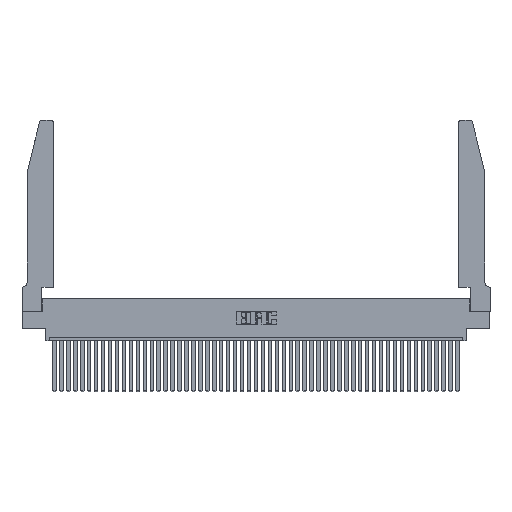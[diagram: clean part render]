
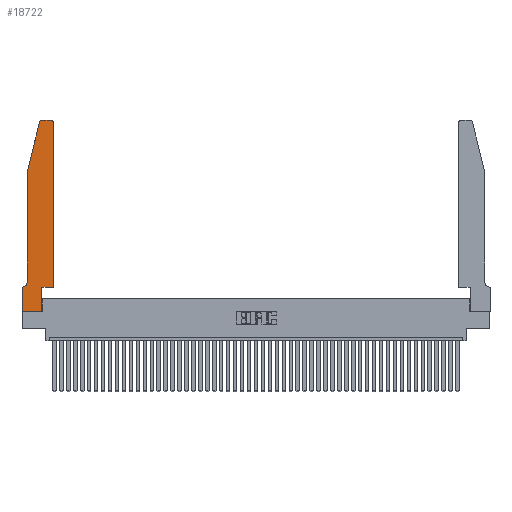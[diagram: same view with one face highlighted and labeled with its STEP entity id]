
A CAD part, top view. The second image highlights one B-rep face of the part: STEP entity #18722.
In plain terms, the highlighted planar face has unit normal (0, 0, 1).
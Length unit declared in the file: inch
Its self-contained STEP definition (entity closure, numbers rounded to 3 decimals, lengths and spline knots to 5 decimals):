
#283 = ORIENTED_EDGE ( 'NONE', *, *, #8491, .T. ) ;
#313 = CIRCLE ( 'NONE', #10665, 0.03 ) ;
#871 = DIRECTION ( 'NONE',  ( 0., 1., 0. ) ) ;
#1090 = AXIS2_PLACEMENT_3D ( 'NONE', #26872, #19271, #1280 ) ;
#1280 = DIRECTION ( 'NONE',  ( -1., 0., 0. ) ) ;
#1536 = CARTESIAN_POINT ( 'NONE',  ( 0.284, 2.72, 0.37 ) ) ;
#1584 = CARTESIAN_POINT ( 'NONE',  ( 0.0755, 2., 0.37 ) ) ;
#2343 = VERTEX_POINT ( 'NONE', #5293 ) ;
#2633 = LINE ( 'NONE', #21457, #19011 ) ;
#3047 = VECTOR ( 'NONE', #44415, 39.37008 ) ;
#3525 = CARTESIAN_POINT ( 'NONE',  ( 0.4505, 0.35, 0.37 ) ) ;
#4507 = EDGE_CURVE ( 'NONE', #11555, #20846, #2633, .T. ) ;
#5060 = DIRECTION ( 'NONE',  ( 1., 0., 0. ) ) ;
#5293 = CARTESIAN_POINT ( 'NONE',  ( 0.2865, 0.35, 0.37 ) ) ;
#5360 = ORIENTED_EDGE ( 'NONE', *, *, #40942, .T. ) ;
#5952 = EDGE_CURVE ( 'NONE', #9379, #37491, #46015, .T. ) ;
#7135 = CARTESIAN_POINT ( 'NONE',  ( 0.0755, 0.42, 0.37 ) ) ;
#7204 = CARTESIAN_POINT ( 'NONE',  ( 0.4505, 0.35, 0.37 ) ) ;
#7274 = EDGE_CURVE ( 'NONE', #20846, #2343, #31733, .T. ) ;
#7823 = VECTOR ( 'NONE', #12005, 39.37008 ) ;
#8034 = CARTESIAN_POINT ( 'NONE',  ( 0.0755, 2., 0.37 ) ) ;
#8142 = LINE ( 'NONE', #18958, #3047 ) ;
#8491 = EDGE_CURVE ( 'NONE', #11571, #30345, #36037, .T. ) ;
#9094 = LINE ( 'NONE', #40212, #46396 ) ;
#9171 = VERTEX_POINT ( 'NONE', #32146 ) ;
#9379 = VERTEX_POINT ( 'NONE', #26579 ) ;
#10449 = EDGE_CURVE ( 'NONE', #13111, #12483, #8142, .T. ) ;
#10665 = AXIS2_PLACEMENT_3D ( 'NONE', #25109, #39788, #43421 ) ;
#11555 = VERTEX_POINT ( 'NONE', #32080 ) ;
#11571 = VERTEX_POINT ( 'NONE', #43424 ) ;
#12005 = DIRECTION ( 'NONE',  ( 0., -1., 0. ) ) ;
#12114 = VECTOR ( 'NONE', #27587, 39.37008 ) ;
#12470 = PLANE ( 'NONE',  #38054 ) ;
#12483 = VERTEX_POINT ( 'NONE', #39222 ) ;
#12697 = LINE ( 'NONE', #19824, #12114 ) ;
#12768 = CARTESIAN_POINT ( 'NONE',  ( 0.284, 2.75, 0.37 ) ) ;
#12787 = ORIENTED_EDGE ( 'NONE', *, *, #10449, .T. ) ;
#13067 = VERTEX_POINT ( 'NONE', #31155 ) ;
#13111 = VERTEX_POINT ( 'NONE', #13577 ) ;
#13577 = CARTESIAN_POINT ( 'NONE',  ( 0.0055, 0.35, 0.37 ) ) ;
#15558 = LINE ( 'NONE', #8034, #38167 ) ;
#17990 = DIRECTION ( 'NONE',  ( 1., 0., 0. ) ) ;
#18722 = ADVANCED_FACE ( 'NONE', ( #31965 ), #12470, .T. ) ;
#18958 = CARTESIAN_POINT ( 'NONE',  ( 0.0755, 0.35, 0.37 ) ) ;
#19011 = VECTOR ( 'NONE', #17990, 39.37008 ) ;
#19051 = ORIENTED_EDGE ( 'NONE', *, *, #35334, .T. ) ;
#19209 = EDGE_CURVE ( 'NONE', #13067, #11571, #15558, .T. ) ;
#19271 = DIRECTION ( 'NONE',  ( 0., 0., -1. ) ) ;
#19824 = CARTESIAN_POINT ( 'NONE',  ( 0., 0., 0.37 ) ) ;
#20846 = VERTEX_POINT ( 'NONE', #46576 ) ;
#21360 = EDGE_CURVE ( 'NONE', #12483, #11555, #12697, .T. ) ;
#21457 = CARTESIAN_POINT ( 'NONE',  ( 0., 0., 0.37 ) ) ;
#21843 = ORIENTED_EDGE ( 'NONE', *, *, #7274, .T. ) ;
#22982 = EDGE_LOOP ( 'NONE', ( #23154, #35315, #29236, #283, #44644, #12787, #43245, #35074, #21843, #19051, #5360, #32032 ) ) ;
#23154 = ORIENTED_EDGE ( 'NONE', *, *, #5952, .T. ) ;
#23184 = DIRECTION ( 'NONE',  ( -1., 0., 0. ) ) ;
#23235 = EDGE_CURVE ( 'NONE', #37491, #13067, #27174, .T. ) ;
#23344 = CARTESIAN_POINT ( 'NONE',  ( 0.2605, 2.75, 0.37 ) ) ;
#23718 = CIRCLE ( 'NONE', #1090, 0.07 ) ;
#25109 = CARTESIAN_POINT ( 'NONE',  ( 0.4205, 2.72, 0.37 ) ) ;
#26169 = DIRECTION ( 'NONE',  ( -0.239, -0.971, 0. ) ) ;
#26535 = LINE ( 'NONE', #7204, #31618 ) ;
#26579 = CARTESIAN_POINT ( 'NONE',  ( 0.4205, 2.75, 0.37 ) ) ;
#26820 = EDGE_CURVE ( 'NONE', #9171, #9379, #313, .T. ) ;
#26872 = CARTESIAN_POINT ( 'NONE',  ( 0.0055, 0.42, 0.37 ) ) ;
#27174 = CIRCLE ( 'NONE', #39029, 0.03 ) ;
#27587 = DIRECTION ( 'NONE',  ( 0., -1., 0. ) ) ;
#29236 = ORIENTED_EDGE ( 'NONE', *, *, #19209, .T. ) ;
#30038 = CARTESIAN_POINT ( 'NONE',  ( 0.2865, 0.35, 0.37 ) ) ;
#30345 = VERTEX_POINT ( 'NONE', #7135 ) ;
#30650 = CARTESIAN_POINT ( 'NONE',  ( 0., 0.35, 0.37 ) ) ;
#31155 = CARTESIAN_POINT ( 'NONE',  ( 0.25487, 2.72718, 0.37 ) ) ;
#31618 = VECTOR ( 'NONE', #36078, 39.37008 ) ;
#31733 = LINE ( 'NONE', #30038, #40755 ) ;
#31965 = FACE_OUTER_BOUND ( 'NONE', #22982, .T. ) ;
#32032 = ORIENTED_EDGE ( 'NONE', *, *, #26820, .T. ) ;
#32080 = CARTESIAN_POINT ( 'NONE',  ( 0., 0., 0.37 ) ) ;
#32146 = CARTESIAN_POINT ( 'NONE',  ( 0.4505, 2.72, 0.37 ) ) ;
#34430 = DIRECTION ( 'NONE',  ( 0., 0., 1. ) ) ;
#35074 = ORIENTED_EDGE ( 'NONE', *, *, #4507, .T. ) ;
#35315 = ORIENTED_EDGE ( 'NONE', *, *, #23235, .T. ) ;
#35334 = EDGE_CURVE ( 'NONE', #2343, #37176, #26535, .T. ) ;
#36037 = LINE ( 'NONE', #1584, #7823 ) ;
#36078 = DIRECTION ( 'NONE',  ( 1., 0., 0. ) ) ;
#37176 = VERTEX_POINT ( 'NONE', #3525 ) ;
#37491 = VERTEX_POINT ( 'NONE', #12768 ) ;
#38052 = DIRECTION ( 'NONE',  ( 1., 0., 0. ) ) ;
#38054 = AXIS2_PLACEMENT_3D ( 'NONE', #30650, #34430, #38052 ) ;
#38167 = VECTOR ( 'NONE', #26169, 39.37008 ) ;
#39029 = AXIS2_PLACEMENT_3D ( 'NONE', #1536, #41184, #5060 ) ;
#39192 = VECTOR ( 'NONE', #23184, 39.37008 ) ;
#39222 = CARTESIAN_POINT ( 'NONE',  ( 0., 0.35, 0.37 ) ) ;
#39788 = DIRECTION ( 'NONE',  ( 0., 0., 1. ) ) ;
#40212 = CARTESIAN_POINT ( 'NONE',  ( 0.4505, 0.35, 0.37 ) ) ;
#40755 = VECTOR ( 'NONE', #44387, 39.37008 ) ;
#40942 = EDGE_CURVE ( 'NONE', #37176, #9171, #9094, .T. ) ;
#41184 = DIRECTION ( 'NONE',  ( 0., 0., 1. ) ) ;
#41703 = EDGE_CURVE ( 'NONE', #30345, #13111, #23718, .T. ) ;
#43245 = ORIENTED_EDGE ( 'NONE', *, *, #21360, .T. ) ;
#43421 = DIRECTION ( 'NONE',  ( 1., 0., 0. ) ) ;
#43424 = CARTESIAN_POINT ( 'NONE',  ( 0.0755, 2., 0.37 ) ) ;
#44387 = DIRECTION ( 'NONE',  ( 0., 1., 0. ) ) ;
#44415 = DIRECTION ( 'NONE',  ( -1., 0., 0. ) ) ;
#44644 = ORIENTED_EDGE ( 'NONE', *, *, #41703, .T. ) ;
#46015 = LINE ( 'NONE', #23344, #39192 ) ;
#46396 = VECTOR ( 'NONE', #871, 39.37008 ) ;
#46576 = CARTESIAN_POINT ( 'NONE',  ( 0.2865, 0., 0.37 ) ) ;
